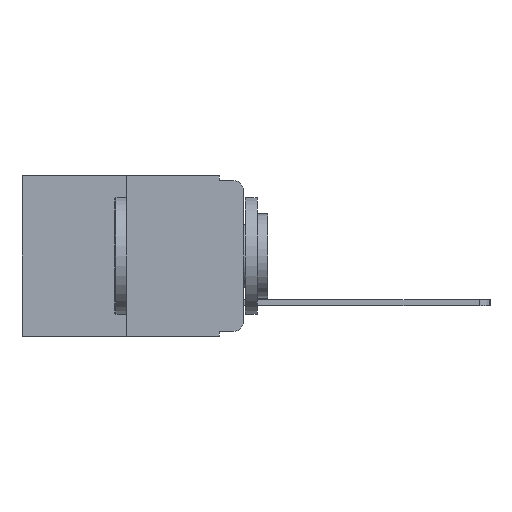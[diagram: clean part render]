
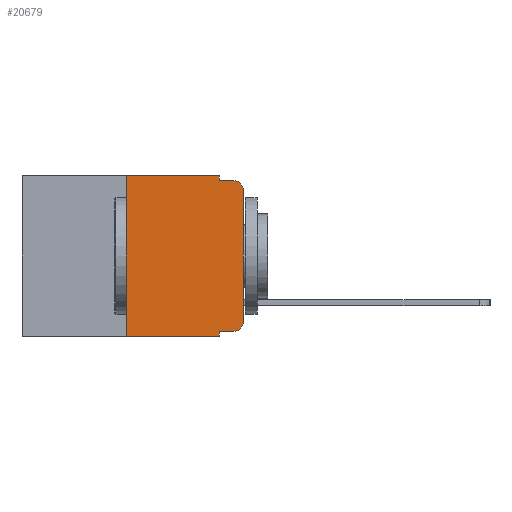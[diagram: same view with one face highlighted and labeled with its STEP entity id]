
A CAD part, left-side view. The second image highlights one B-rep face of the part: STEP entity #20679.
In plain terms, the highlighted planar face has unit normal (-1, 0, 0).
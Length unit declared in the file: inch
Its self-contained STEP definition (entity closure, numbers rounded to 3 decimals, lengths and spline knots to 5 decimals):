
#192 = LINE ( 'NONE', #6033, #9712 ) ;
#525 = CARTESIAN_POINT ( 'NONE',  ( 0., 0.25, 0. ) ) ;
#1076 = EDGE_LOOP ( 'NONE', ( #4384, #7873, #15449, #18513, #15149, #18265, #6714, #11778, #21689, #7697 ) ) ;
#1350 = DIRECTION ( 'NONE',  ( 0., 0., -1. ) ) ;
#1501 = CARTESIAN_POINT ( 'NONE',  ( 0., 0.051, -0.333 ) ) ;
#1742 = VECTOR ( 'NONE', #9270, 39.37008 ) ;
#2083 = CARTESIAN_POINT ( 'NONE',  ( 0., 0.02, -0.333 ) ) ;
#2233 = VERTEX_POINT ( 'NONE', #6533 ) ;
#2838 = EDGE_CURVE ( 'NONE', #19001, #3492, #12545, .T. ) ;
#2926 = LINE ( 'NONE', #22261, #18948 ) ;
#3492 = VERTEX_POINT ( 'NONE', #5212 ) ;
#3758 = LINE ( 'NONE', #8882, #23699 ) ;
#4062 = VERTEX_POINT ( 'NONE', #7032 ) ;
#4384 = ORIENTED_EDGE ( 'NONE', *, *, #20719, .T. ) ;
#4533 = CARTESIAN_POINT ( 'NONE',  ( 0., 0.25, 0. ) ) ;
#4636 = CARTESIAN_POINT ( 'NONE',  ( 0., 0., -0.03 ) ) ;
#5212 = CARTESIAN_POINT ( 'NONE',  ( 0., 0.051, 0. ) ) ;
#5499 = CARTESIAN_POINT ( 'NONE',  ( 0., 0.02, -0.03 ) ) ;
#5732 = EDGE_CURVE ( 'NONE', #12159, #6338, #2926, .T. ) ;
#6033 = CARTESIAN_POINT ( 'NONE',  ( 0., 0.473, -0.343 ) ) ;
#6338 = VERTEX_POINT ( 'NONE', #2083 ) ;
#6533 = CARTESIAN_POINT ( 'NONE',  ( 0., 0.25, -0.343 ) ) ;
#6714 = ORIENTED_EDGE ( 'NONE', *, *, #9924, .T. ) ;
#7032 = CARTESIAN_POINT ( 'NONE',  ( 0., 0.051, -0.01 ) ) ;
#7092 = VECTOR ( 'NONE', #11832, 39.37008 ) ;
#7508 = DIRECTION ( 'NONE',  ( 0., 0., -1. ) ) ;
#7598 = PLANE ( 'NONE',  #8166 ) ;
#7697 = ORIENTED_EDGE ( 'NONE', *, *, #25484, .T. ) ;
#7873 = ORIENTED_EDGE ( 'NONE', *, *, #20646, .T. ) ;
#8016 = DIRECTION ( 'NONE',  ( 0., -1., 0. ) ) ;
#8097 = AXIS2_PLACEMENT_3D ( 'NONE', #11688, #25402, #13707 ) ;
#8157 = VERTEX_POINT ( 'NONE', #20263 ) ;
#8166 = AXIS2_PLACEMENT_3D ( 'NONE', #11563, #25379, #13677 ) ;
#8372 = CARTESIAN_POINT ( 'NONE',  ( 0., 0., -0.313 ) ) ;
#8882 = CARTESIAN_POINT ( 'NONE',  ( 0., 0.051, 0. ) ) ;
#9270 = DIRECTION ( 'NONE',  ( 0., -1., 0. ) ) ;
#9441 = EDGE_CURVE ( 'NONE', #2233, #19001, #15734, .T. ) ;
#9712 = VECTOR ( 'NONE', #8016, 39.37008 ) ;
#9924 = EDGE_CURVE ( 'NONE', #2233, #8157, #192, .T. ) ;
#10375 = DIRECTION ( 'NONE',  ( 0., -1., 0. ) ) ;
#10377 = CARTESIAN_POINT ( 'NONE',  ( 0., 0.051, -0.01 ) ) ;
#10827 = CARTESIAN_POINT ( 'NONE',  ( 0., 0.02, -0.01 ) ) ;
#11563 = CARTESIAN_POINT ( 'NONE',  ( 0., 0.473, 0. ) ) ;
#11688 = CARTESIAN_POINT ( 'NONE',  ( 0., 0.02, -0.313 ) ) ;
#11778 = ORIENTED_EDGE ( 'NONE', *, *, #15543, .F. ) ;
#11832 = DIRECTION ( 'NONE',  ( 0., 0., 1. ) ) ;
#12159 = VERTEX_POINT ( 'NONE', #1501 ) ;
#12257 = VECTOR ( 'NONE', #20292, 39.37008 ) ;
#12545 = LINE ( 'NONE', #23166, #1742 ) ;
#13072 = VERTEX_POINT ( 'NONE', #4636 ) ;
#13677 = DIRECTION ( 'NONE',  ( 0., 0., -1. ) ) ;
#13707 = DIRECTION ( 'NONE',  ( 0., 0., -1. ) ) ;
#13782 = EDGE_CURVE ( 'NONE', #3492, #4062, #3758, .T. ) ;
#14094 = CIRCLE ( 'NONE', #8097, 0.02 ) ;
#14556 = EDGE_CURVE ( 'NONE', #4062, #21061, #22147, .T. ) ;
#15149 = ORIENTED_EDGE ( 'NONE', *, *, #2838, .F. ) ;
#15449 = ORIENTED_EDGE ( 'NONE', *, *, #14556, .F. ) ;
#15543 = EDGE_CURVE ( 'NONE', #12159, #8157, #19645, .T. ) ;
#15734 = LINE ( 'NONE', #4533, #25462 ) ;
#15842 = VERTEX_POINT ( 'NONE', #8372 ) ;
#17752 = CARTESIAN_POINT ( 'NONE',  ( 0., 0., 0. ) ) ;
#18265 = ORIENTED_EDGE ( 'NONE', *, *, #9441, .F. ) ;
#18349 = CIRCLE ( 'NONE', #24576, 0.02 ) ;
#18513 = ORIENTED_EDGE ( 'NONE', *, *, #13782, .F. ) ;
#18948 = VECTOR ( 'NONE', #10375, 39.37008 ) ;
#19001 = VERTEX_POINT ( 'NONE', #525 ) ;
#19461 = DIRECTION ( 'NONE',  ( -1., 0., 0. ) ) ;
#19645 = LINE ( 'NONE', #21353, #23611 ) ;
#20263 = CARTESIAN_POINT ( 'NONE',  ( 0., 0.051, -0.343 ) ) ;
#20292 = DIRECTION ( 'NONE',  ( 0., -1., 0. ) ) ;
#20501 = DIRECTION ( 'NONE',  ( 0., 0., 1. ) ) ;
#20646 = EDGE_CURVE ( 'NONE', #13072, #21061, #18349, .T. ) ;
#20679 = ADVANCED_FACE ( 'NONE', ( #22961 ), #7598, .F. ) ;
#20719 = EDGE_CURVE ( 'NONE', #15842, #13072, #21708, .T. ) ;
#20902 = DIRECTION ( 'NONE',  ( 0., 0., -1. ) ) ;
#21061 = VERTEX_POINT ( 'NONE', #10827 ) ;
#21353 = CARTESIAN_POINT ( 'NONE',  ( 0., 0.051, 0. ) ) ;
#21689 = ORIENTED_EDGE ( 'NONE', *, *, #5732, .T. ) ;
#21708 = LINE ( 'NONE', #17752, #7092 ) ;
#22147 = LINE ( 'NONE', #10377, #12257 ) ;
#22261 = CARTESIAN_POINT ( 'NONE',  ( 0., 0.051, -0.333 ) ) ;
#22961 = FACE_OUTER_BOUND ( 'NONE', #1076, .T. ) ;
#23166 = CARTESIAN_POINT ( 'NONE',  ( 0., 0.473, 0. ) ) ;
#23611 = VECTOR ( 'NONE', #1350, 39.37008 ) ;
#23699 = VECTOR ( 'NONE', #20902, 39.37008 ) ;
#24576 = AXIS2_PLACEMENT_3D ( 'NONE', #5499, #19461, #7508 ) ;
#25379 = DIRECTION ( 'NONE',  ( 1., 0., 0. ) ) ;
#25402 = DIRECTION ( 'NONE',  ( -1., 0., 0. ) ) ;
#25462 = VECTOR ( 'NONE', #20501, 39.37008 ) ;
#25484 = EDGE_CURVE ( 'NONE', #6338, #15842, #14094, .T. ) ;
